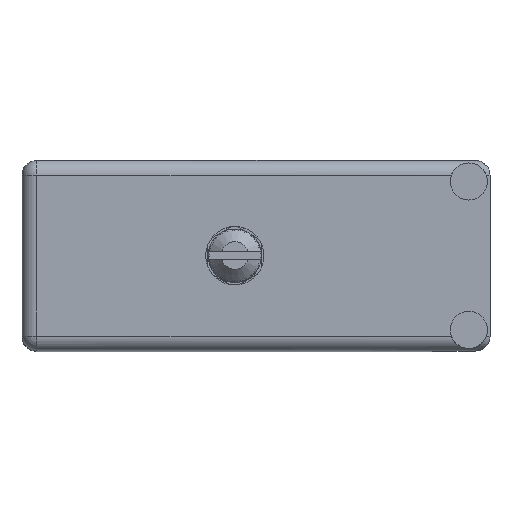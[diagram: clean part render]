
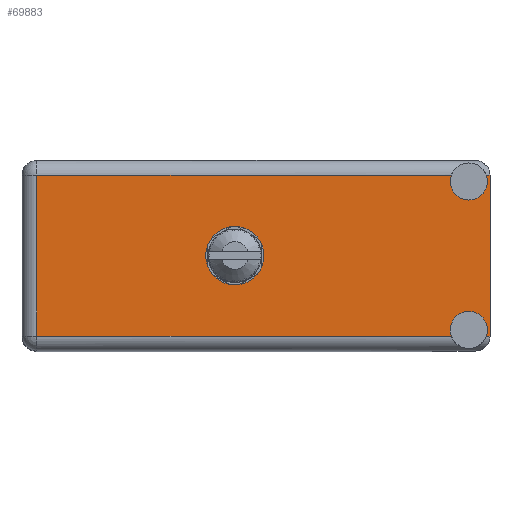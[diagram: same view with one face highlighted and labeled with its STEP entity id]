
A CAD part, top view. The second image highlights one B-rep face of the part: STEP entity #69883.
In plain terms, the highlighted face is planar.
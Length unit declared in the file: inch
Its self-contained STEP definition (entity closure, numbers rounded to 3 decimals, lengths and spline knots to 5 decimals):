
#403 = CARTESIAN_POINT ( 'NONE',  ( 0., 1.566, -0.829 ) ) ;
#1244 = DIRECTION ( 'NONE',  ( 0., 1., 0. ) ) ;
#1613 = CARTESIAN_POINT ( 'NONE',  ( 0., 1.566, -0.899 ) ) ;
#3213 = DIRECTION ( 'NONE',  ( 0., 1., 0. ) ) ;
#3773 = VERTEX_POINT ( 'NONE', #112570 ) ;
#3884 = VERTEX_POINT ( 'NONE', #104012 ) ;
#5202 = CARTESIAN_POINT ( 'NONE',  ( 2.02562, 1.566, -0.07 ) ) ;
#6243 = LINE ( 'NONE', #40550, #79443 ) ;
#10616 = CARTESIAN_POINT ( 'NONE',  ( 2.108, 1.566, -0.0995 ) ) ;
#11189 = DIRECTION ( 'NONE',  ( 0., 1., 0. ) ) ;
#11454 = AXIS2_PLACEMENT_3D ( 'NONE', #64998, #20419, #37560 ) ;
#11938 = EDGE_CURVE ( 'NONE', #83409, #61877, #65098, .T. ) ;
#14386 = DIRECTION ( 'NONE',  ( 0., 0., 1. ) ) ;
#15927 = VERTEX_POINT ( 'NONE', #108027 ) ;
#18734 = CIRCLE ( 'NONE', #11454, 0.0875 ) ;
#18911 = CARTESIAN_POINT ( 'NONE',  ( 0.07, 1.566, -0.829 ) ) ;
#19518 = EDGE_CURVE ( 'NONE', #104011, #77432, #73538, .T. ) ;
#19902 = EDGE_CURVE ( 'NONE', #28882, #83409, #88928, .T. ) ;
#20419 = DIRECTION ( 'NONE',  ( 0., 1., 0. ) ) ;
#21305 = DIRECTION ( 'NONE',  ( 0., 0., 1. ) ) ;
#21665 = CARTESIAN_POINT ( 'NONE',  ( 0.07, 1.566, -0.899 ) ) ;
#21996 = CARTESIAN_POINT ( 'NONE',  ( 1.004, 1.566, -0.312 ) ) ;
#22069 = AXIS2_PLACEMENT_3D ( 'NONE', #47419, #39369, #89103 ) ;
#23220 = EDGE_CURVE ( 'NONE', #106381, #44532, #102684, .T. ) ;
#23652 = LINE ( 'NONE', #60217, #111831 ) ;
#24202 = AXIS2_PLACEMENT_3D ( 'NONE', #105176, #1244, #44124 ) ;
#25264 = VECTOR ( 'NONE', #21305, 39.37008 ) ;
#28882 = VERTEX_POINT ( 'NONE', #34824 ) ;
#29079 = CARTESIAN_POINT ( 'NONE',  ( 1.004, 1.566, -0.587 ) ) ;
#33230 = EDGE_LOOP ( 'NONE', ( #56405, #82238, #91915, #84613, #53914, #80678, #110470, #43552, #83892, #63075 ) ) ;
#33917 = DIRECTION ( 'NONE',  ( 1., 0., 0. ) ) ;
#34824 = CARTESIAN_POINT ( 'NONE',  ( 2.02562, 1.566, -0.829 ) ) ;
#35684 = EDGE_CURVE ( 'NONE', #3884, #52484, #18734, .T. ) ;
#36244 = ORIENTED_EDGE ( 'NONE', *, *, #23220, .F. ) ;
#36388 = CARTESIAN_POINT ( 'NONE',  ( 0.07, 1.566, -0.07 ) ) ;
#36456 = DIRECTION ( 'NONE',  ( 0., 1., 0. ) ) ;
#37560 = DIRECTION ( 'NONE',  ( 0., 0., 1. ) ) ;
#39369 = DIRECTION ( 'NONE',  ( 0., 1., 0. ) ) ;
#40550 = CARTESIAN_POINT ( 'NONE',  ( 2.208, 1.566, -0.07 ) ) ;
#43552 = ORIENTED_EDGE ( 'NONE', *, *, #100162, .F. ) ;
#44124 = DIRECTION ( 'NONE',  ( 0., 0., 1. ) ) ;
#44532 = VERTEX_POINT ( 'NONE', #29079 ) ;
#45072 = FACE_OUTER_BOUND ( 'NONE', #33230, .T. ) ;
#46463 = LINE ( 'NONE', #90416, #25264 ) ;
#47419 = CARTESIAN_POINT ( 'NONE',  ( 2.108, 1.566, -0.7995 ) ) ;
#52484 = VERTEX_POINT ( 'NONE', #71842 ) ;
#53914 = ORIENTED_EDGE ( 'NONE', *, *, #70243, .F. ) ;
#56405 = ORIENTED_EDGE ( 'NONE', *, *, #102769, .T. ) ;
#56519 = DIRECTION ( 'NONE',  ( 0., 0., 1. ) ) ;
#58264 = VECTOR ( 'NONE', #56519, 39.37008 ) ;
#58822 = EDGE_LOOP ( 'NONE', ( #36244, #85655 ) ) ;
#59506 = CARTESIAN_POINT ( 'NONE',  ( 1.004, 1.566, -0.4495 ) ) ;
#60217 = CARTESIAN_POINT ( 'NONE',  ( 2.208, 1.566, -0.07 ) ) ;
#60939 = VERTEX_POINT ( 'NONE', #93571 ) ;
#61877 = VERTEX_POINT ( 'NONE', #36388 ) ;
#63075 = ORIENTED_EDGE ( 'NONE', *, *, #11938, .T. ) ;
#64998 = CARTESIAN_POINT ( 'NONE',  ( 2.108, 1.566, -0.7995 ) ) ;
#65098 = LINE ( 'NONE', #21665, #58264 ) ;
#65424 = AXIS2_PLACEMENT_3D ( 'NONE', #1613, #36456, #79354 ) ;
#69883 = ADVANCED_FACE ( 'NONE', ( #70806, #45072 ), #100790, .T. ) ;
#70243 = EDGE_CURVE ( 'NONE', #15927, #60939, #46463, .T. ) ;
#70715 = DIRECTION ( 'NONE',  ( -1., 0., 0. ) ) ;
#70806 = FACE_BOUND ( 'NONE', #58822, .T. ) ;
#71842 = CARTESIAN_POINT ( 'NONE',  ( 2.19038, 1.566, -0.829 ) ) ;
#73538 = CIRCLE ( 'NONE', #24202, 0.0875 ) ;
#76062 = AXIS2_PLACEMENT_3D ( 'NONE', #10616, #11189, #88347 ) ;
#77432 = VERTEX_POINT ( 'NONE', #5202 ) ;
#78391 = EDGE_CURVE ( 'NONE', #44532, #106381, #92051, .T. ) ;
#79354 = DIRECTION ( 'NONE',  ( 0., 0., 1. ) ) ;
#79443 = VECTOR ( 'NONE', #110172, 39.37008 ) ;
#80678 = ORIENTED_EDGE ( 'NONE', *, *, #88195, .T. ) ;
#82238 = ORIENTED_EDGE ( 'NONE', *, *, #19518, .F. ) ;
#82339 = CIRCLE ( 'NONE', #22069, 0.0875 ) ;
#83342 = CIRCLE ( 'NONE', #76062, 0.0875 ) ;
#83409 = VERTEX_POINT ( 'NONE', #18911 ) ;
#83581 = EDGE_CURVE ( 'NONE', #3773, #60939, #6243, .T. ) ;
#83892 = ORIENTED_EDGE ( 'NONE', *, *, #19902, .T. ) ;
#84481 = AXIS2_PLACEMENT_3D ( 'NONE', #108252, #3213, #109383 ) ;
#84613 = ORIENTED_EDGE ( 'NONE', *, *, #83581, .T. ) ;
#85655 = ORIENTED_EDGE ( 'NONE', *, *, #78391, .F. ) ;
#86292 = VECTOR ( 'NONE', #99730, 39.37008 ) ;
#86690 = LINE ( 'NONE', #403, #90660 ) ;
#87225 = EDGE_CURVE ( 'NONE', #3773, #104011, #83342, .T. ) ;
#88195 = EDGE_CURVE ( 'NONE', #15927, #52484, #86690, .T. ) ;
#88347 = DIRECTION ( 'NONE',  ( 0., 0., 1. ) ) ;
#88928 = LINE ( 'NONE', #107703, #86292 ) ;
#89103 = DIRECTION ( 'NONE',  ( 0., 0., 1. ) ) ;
#90416 = CARTESIAN_POINT ( 'NONE',  ( 2.208, 1.566, 0. ) ) ;
#90660 = VECTOR ( 'NONE', #70715, 39.37008 ) ;
#91915 = ORIENTED_EDGE ( 'NONE', *, *, #87225, .F. ) ;
#92051 = CIRCLE ( 'NONE', #103028, 0.1375 ) ;
#93571 = CARTESIAN_POINT ( 'NONE',  ( 2.208, 1.566, -0.07 ) ) ;
#99730 = DIRECTION ( 'NONE',  ( -1., 0., 0. ) ) ;
#100162 = EDGE_CURVE ( 'NONE', #28882, #3884, #82339, .T. ) ;
#100790 = PLANE ( 'NONE',  #65424 ) ;
#100897 = CARTESIAN_POINT ( 'NONE',  ( 2.108, 1.566, -0.187 ) ) ;
#101726 = DIRECTION ( 'NONE',  ( 0., 1., 0. ) ) ;
#102684 = CIRCLE ( 'NONE', #84481, 0.1375 ) ;
#102769 = EDGE_CURVE ( 'NONE', #61877, #77432, #23652, .T. ) ;
#103028 = AXIS2_PLACEMENT_3D ( 'NONE', #59506, #101726, #14386 ) ;
#104011 = VERTEX_POINT ( 'NONE', #100897 ) ;
#104012 = CARTESIAN_POINT ( 'NONE',  ( 2.108, 1.566, -0.712 ) ) ;
#105176 = CARTESIAN_POINT ( 'NONE',  ( 2.108, 1.566, -0.0995 ) ) ;
#106381 = VERTEX_POINT ( 'NONE', #21996 ) ;
#107703 = CARTESIAN_POINT ( 'NONE',  ( 0., 1.566, -0.829 ) ) ;
#108027 = CARTESIAN_POINT ( 'NONE',  ( 2.208, 1.566, -0.829 ) ) ;
#108252 = CARTESIAN_POINT ( 'NONE',  ( 1.004, 1.566, -0.4495 ) ) ;
#109383 = DIRECTION ( 'NONE',  ( 0., 0., 1. ) ) ;
#110172 = DIRECTION ( 'NONE',  ( 1., 0., 0. ) ) ;
#110470 = ORIENTED_EDGE ( 'NONE', *, *, #35684, .F. ) ;
#111831 = VECTOR ( 'NONE', #33917, 39.37008 ) ;
#112570 = CARTESIAN_POINT ( 'NONE',  ( 2.19038, 1.566, -0.07 ) ) ;
